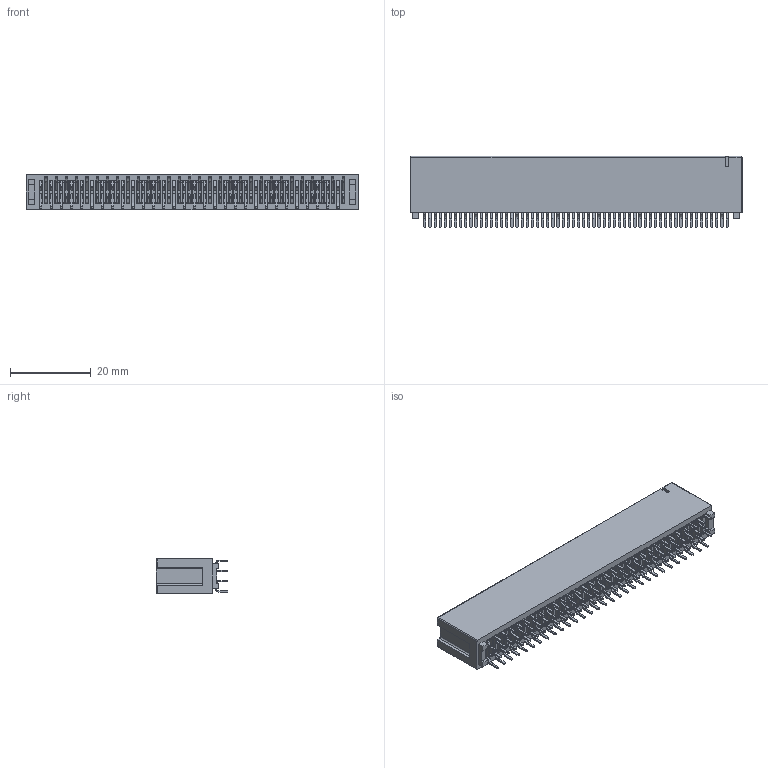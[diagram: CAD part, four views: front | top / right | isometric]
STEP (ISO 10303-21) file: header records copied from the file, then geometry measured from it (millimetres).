
FILE_DESCRIPTION (( 'STEP AP203' ), '1' );
FILE_NAME ('302-120-221-201.STEP', '2024-04-01T19:37:22', ( '' ), ( '' ), 'SwSTEP 2.0', 'SolidWorks 2023', '' );
FILE_SCHEMA (( 'CONFIG_CONTROL_DESIGN' ));
Length unit declared in the file: millimetre
Products named in the file (4): HSG_Vertical HSG; 302-120-221-201; Contact_302-290-X21 (2); Contact_302-290-X21 (1)
Assembly tree (121 placements, depth 2):
  302-120-221-201
    HSG_Vertical HSG
    Contact_302-290-X21 (2)  x60
    Contact_302-290-X21 (1)  x60
Bounding box: 82.3 x 17.63 x 8.88 mm (x, y, z)
Volume: 6254.1 mm3; surface area: 17951 mm2
Topology: 121 solids, 121 shells, 5526 faces, 16248 edges, 10664 vertices
Faces by surface type: plane 4069, cylinder 1213, bspline 240, sphere 4
Entity records: 46136 total; most frequent: ORIENTED_EDGE 7944, CARTESIAN_POINT 7882, DIRECTION 6354, EDGE_CURVE 3972, VECTOR 3898, LINE 3898, VERTEX_POINT 2640, AXIS2_PLACEMENT_3D 1228
